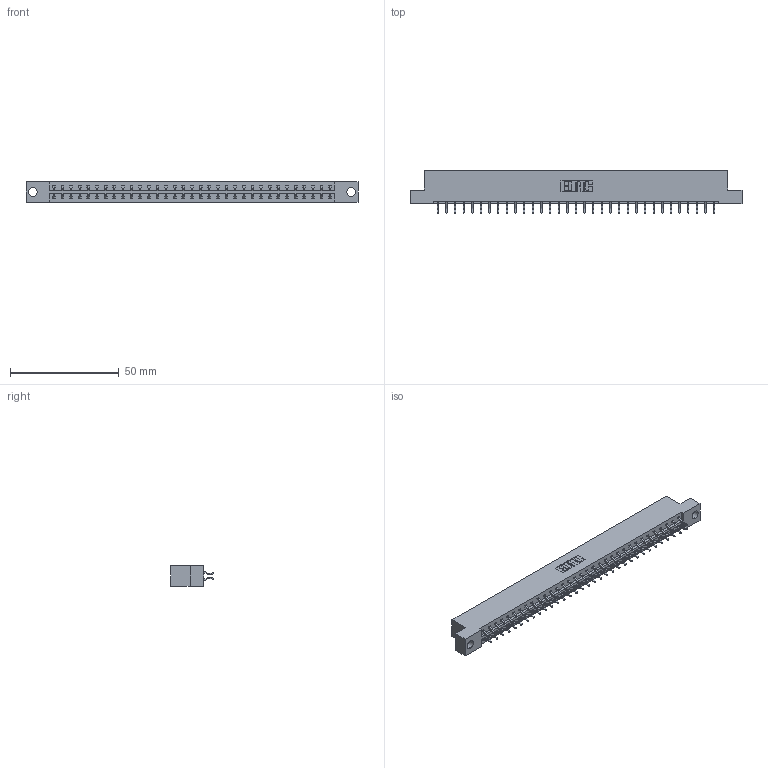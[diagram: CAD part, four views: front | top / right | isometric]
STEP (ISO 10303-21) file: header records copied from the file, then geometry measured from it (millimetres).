
FILE_DESCRIPTION (( 'STEP AP203' ), '1' );
FILE_NAME ('333-066-556-204.STEP', '2018-08-04T11:53:50', ( '' ), ( '' ), 'SwSTEP 2.0', 'SolidWorks 2016', '' );
FILE_SCHEMA (( 'CONFIG_CONTROL_DESIGN' ));
Length unit declared in the file: inch
Products named in the file (3): 333 Part_Flush - .156 Dia - TH; 345-292-001_556 Tail; 333-066-556-204
Assembly tree (67 placements, depth 2):
  333-066-556-204
    333 Part_Flush - .156 Dia - TH
    345-292-001_556 Tail  x66
Bounding box: 152.3 x 19.57 x 9.4 mm (x, y, z)
Volume: 15374.2 mm3; surface area: 17813.7 mm2
Topology: 67 solids, 67 shells, 3942 faces, 11729 edges, 7730 vertices
Faces by surface type: plane 2710, cylinder 1232
Entity records: 22617 total; most frequent: CARTESIAN_POINT 3774, ORIENTED_EDGE 3698, DIRECTION 3229, EDGE_CURVE 1849, VECTOR 1713, LINE 1713, VERTEX_POINT 1230, AXIS2_PLACEMENT_3D 758
